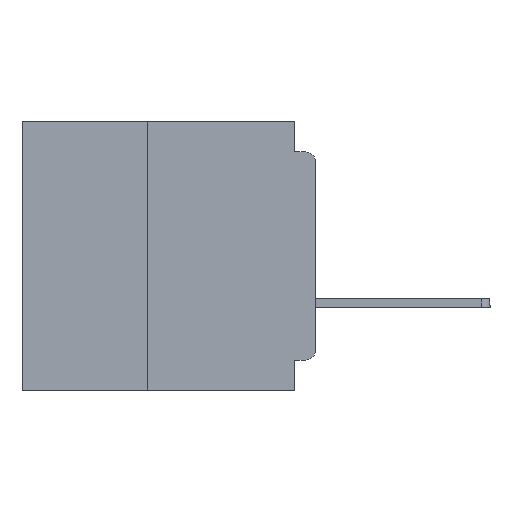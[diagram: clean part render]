
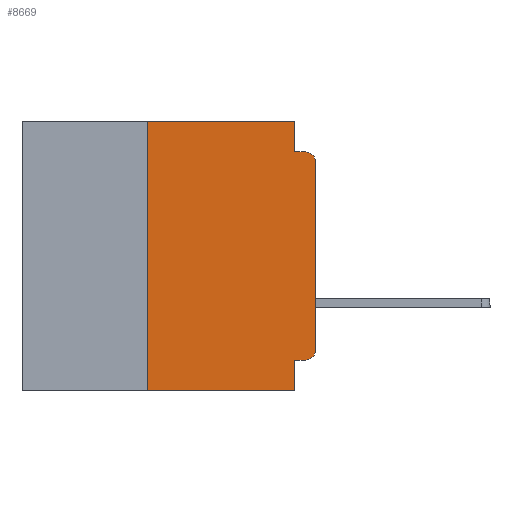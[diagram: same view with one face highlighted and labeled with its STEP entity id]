
A CAD part, left-side view. The second image highlights one B-rep face of the part: STEP entity #8669.
In plain terms, the highlighted planar face has unit normal (-1, 0, 0).
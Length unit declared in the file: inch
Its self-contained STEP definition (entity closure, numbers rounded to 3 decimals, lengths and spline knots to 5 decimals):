
#400 = DIRECTION ( 'NONE',  ( 0., -1., 0. ) ) ;
#875 = EDGE_CURVE ( 'NONE', #52029, #53286, #5725, .T. ) ;
#3660 = DIRECTION ( 'NONE',  ( 0., -1., 0. ) ) ;
#5180 = CARTESIAN_POINT ( 'NONE',  ( 0., 0.031, -0.355 ) ) ;
#5725 = LINE ( 'NONE', #29472, #39509 ) ;
#6426 = AXIS2_PLACEMENT_3D ( 'NONE', #32911, #7549, #37198 ) ;
#6802 = LINE ( 'NONE', #12403, #28022 ) ;
#6838 = CARTESIAN_POINT ( 'NONE',  ( 0., 0.031, 0. ) ) ;
#7549 = DIRECTION ( 'NONE',  ( -1., 0., 0. ) ) ;
#7886 = CARTESIAN_POINT ( 'NONE',  ( 0., 0.25, -0.4 ) ) ;
#8139 = CARTESIAN_POINT ( 'NONE',  ( 0., 0., -0.06 ) ) ;
#8669 = ADVANCED_FACE ( 'NONE', ( #47451 ), #34049, .F. ) ;
#9043 = ORIENTED_EDGE ( 'NONE', *, *, #26398, .F. ) ;
#10396 = CARTESIAN_POINT ( 'NONE',  ( 0., 0.031, -0.4 ) ) ;
#10813 = VECTOR ( 'NONE', #41294, 39.37008 ) ;
#11023 = CARTESIAN_POINT ( 'NONE',  ( 0., 0.25, -0.4 ) ) ;
#11491 = AXIS2_PLACEMENT_3D ( 'NONE', #42548, #46703, #21492 ) ;
#11661 = CARTESIAN_POINT ( 'NONE',  ( 0., 0.015, -0.355 ) ) ;
#12283 = CIRCLE ( 'NONE', #6426, 0.015 ) ;
#12403 = CARTESIAN_POINT ( 'NONE',  ( 0., 0., -0.045 ) ) ;
#12700 = AXIS2_PLACEMENT_3D ( 'NONE', #38145, #12753, #42401 ) ;
#12753 = DIRECTION ( 'NONE',  ( -1., 0., 0. ) ) ;
#13275 = LINE ( 'NONE', #24761, #35886 ) ;
#14839 = ORIENTED_EDGE ( 'NONE', *, *, #50576, .F. ) ;
#14970 = CARTESIAN_POINT ( 'NONE',  ( 0., 0., 0. ) ) ;
#16971 = CIRCLE ( 'NONE', #12700, 0.015 ) ;
#18045 = CARTESIAN_POINT ( 'NONE',  ( 0., 0.25, 0. ) ) ;
#18070 = LINE ( 'NONE', #11023, #25361 ) ;
#18413 = VECTOR ( 'NONE', #40342, 39.37008 ) ;
#18433 = EDGE_CURVE ( 'NONE', #52720, #51340, #6802, .T. ) ;
#19748 = VERTEX_POINT ( 'NONE', #18045 ) ;
#20327 = VERTEX_POINT ( 'NONE', #26146 ) ;
#20956 = DIRECTION ( 'NONE',  ( 0., -1., 0. ) ) ;
#21492 = DIRECTION ( 'NONE',  ( 0., 0., -1. ) ) ;
#21715 = VERTEX_POINT ( 'NONE', #8139 ) ;
#24761 = CARTESIAN_POINT ( 'NONE',  ( 0., 0.437, 0. ) ) ;
#25361 = VECTOR ( 'NONE', #49243, 39.37008 ) ;
#25412 = EDGE_CURVE ( 'NONE', #38314, #20327, #12283, .T. ) ;
#25789 = CARTESIAN_POINT ( 'NONE',  ( 0., 0.437, -0.4 ) ) ;
#26146 = CARTESIAN_POINT ( 'NONE',  ( 0., 0., -0.34 ) ) ;
#26398 = EDGE_CURVE ( 'NONE', #45026, #52720, #28127, .T. ) ;
#26538 = CARTESIAN_POINT ( 'NONE',  ( 0., 0.031, 0. ) ) ;
#28022 = VECTOR ( 'NONE', #20956, 39.37008 ) ;
#28127 = LINE ( 'NONE', #26538, #49162 ) ;
#28282 = ORIENTED_EDGE ( 'NONE', *, *, #51338, .T. ) ;
#28509 = LINE ( 'NONE', #25789, #50844 ) ;
#29402 = ORIENTED_EDGE ( 'NONE', *, *, #875, .F. ) ;
#29472 = CARTESIAN_POINT ( 'NONE',  ( 0., 0.031, -0.4 ) ) ;
#30862 = CARTESIAN_POINT ( 'NONE',  ( 0., 0.031, -0.045 ) ) ;
#31736 = ORIENTED_EDGE ( 'NONE', *, *, #31847, .T. ) ;
#31847 = EDGE_CURVE ( 'NONE', #20327, #21715, #42234, .T. ) ;
#32062 = LINE ( 'NONE', #37065, #10813 ) ;
#32079 = ORIENTED_EDGE ( 'NONE', *, *, #36676, .F. ) ;
#32652 = ORIENTED_EDGE ( 'NONE', *, *, #37217, .F. ) ;
#32911 = CARTESIAN_POINT ( 'NONE',  ( 0., 0.015, -0.34 ) ) ;
#34049 = PLANE ( 'NONE',  #11491 ) ;
#35886 = VECTOR ( 'NONE', #3660, 39.37008 ) ;
#36676 = EDGE_CURVE ( 'NONE', #38314, #52029, #32062, .T. ) ;
#37065 = CARTESIAN_POINT ( 'NONE',  ( 0., 0., -0.355 ) ) ;
#37198 = DIRECTION ( 'NONE',  ( 0., 0., -1. ) ) ;
#37217 = EDGE_CURVE ( 'NONE', #39549, #19748, #18070, .T. ) ;
#37538 = ORIENTED_EDGE ( 'NONE', *, *, #47749, .T. ) ;
#38145 = CARTESIAN_POINT ( 'NONE',  ( 0., 0.015, -0.06 ) ) ;
#38257 = ORIENTED_EDGE ( 'NONE', *, *, #18433, .F. ) ;
#38314 = VERTEX_POINT ( 'NONE', #11661 ) ;
#39509 = VECTOR ( 'NONE', #42257, 39.37008 ) ;
#39549 = VERTEX_POINT ( 'NONE', #7886 ) ;
#40342 = DIRECTION ( 'NONE',  ( 0., 0., 1. ) ) ;
#41294 = DIRECTION ( 'NONE',  ( 0., 1., 0. ) ) ;
#42234 = LINE ( 'NONE', #14970, #18413 ) ;
#42257 = DIRECTION ( 'NONE',  ( 0., 0., -1. ) ) ;
#42401 = DIRECTION ( 'NONE',  ( 0., 0., -1. ) ) ;
#42548 = CARTESIAN_POINT ( 'NONE',  ( 0., 0.437, 0. ) ) ;
#45026 = VERTEX_POINT ( 'NONE', #6838 ) ;
#46703 = DIRECTION ( 'NONE',  ( 1., 0., 0. ) ) ;
#47451 = FACE_OUTER_BOUND ( 'NONE', #54558, .T. ) ;
#47749 = EDGE_CURVE ( 'NONE', #21715, #51340, #16971, .T. ) ;
#49162 = VECTOR ( 'NONE', #51712, 39.37008 ) ;
#49243 = DIRECTION ( 'NONE',  ( 0., 0., 1. ) ) ;
#50576 = EDGE_CURVE ( 'NONE', #19748, #45026, #13275, .T. ) ;
#50844 = VECTOR ( 'NONE', #400, 39.37008 ) ;
#50991 = CARTESIAN_POINT ( 'NONE',  ( 0., 0.015, -0.045 ) ) ;
#51338 = EDGE_CURVE ( 'NONE', #39549, #53286, #28509, .T. ) ;
#51340 = VERTEX_POINT ( 'NONE', #50991 ) ;
#51712 = DIRECTION ( 'NONE',  ( 0., 0., -1. ) ) ;
#52029 = VERTEX_POINT ( 'NONE', #5180 ) ;
#52720 = VERTEX_POINT ( 'NONE', #30862 ) ;
#53286 = VERTEX_POINT ( 'NONE', #10396 ) ;
#53912 = ORIENTED_EDGE ( 'NONE', *, *, #25412, .T. ) ;
#54558 = EDGE_LOOP ( 'NONE', ( #31736, #37538, #38257, #9043, #14839, #32652, #28282, #29402, #32079, #53912 ) ) ;
